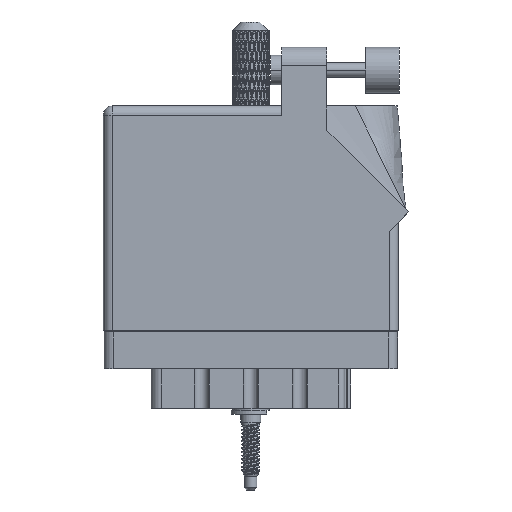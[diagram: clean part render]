
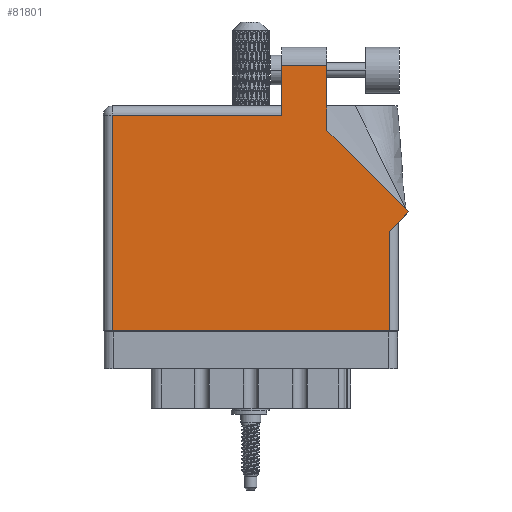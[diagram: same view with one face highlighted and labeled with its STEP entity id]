
A CAD part, front view. The second image highlights one B-rep face of the part: STEP entity #81801.
In plain terms, the highlighted face is planar.
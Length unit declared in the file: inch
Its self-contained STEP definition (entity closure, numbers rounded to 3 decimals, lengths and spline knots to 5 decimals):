
#190 = CARTESIAN_POINT ( 'NONE',  ( 1.524, 1.805, 0. ) ) ;
#552 = CARTESIAN_POINT ( 'NONE',  ( 0., 1.53, 0. ) ) ;
#3980 = ORIENTED_EDGE ( 'NONE', *, *, #29289, .T. ) ;
#4600 = LINE ( 'NONE', #6579, #17549 ) ;
#6579 = CARTESIAN_POINT ( 'NONE',  ( 0., 1.468, 0. ) ) ;
#6887 = DIRECTION ( 'NONE',  ( -0.707, 0.707, 0. ) ) ;
#7116 = DIRECTION ( 'NONE',  ( -1., 0., 0. ) ) ;
#8156 = DIRECTION ( 'NONE',  ( 0., 0., -1. ) ) ;
#11079 = LINE ( 'NONE', #96018, #40867 ) ;
#14745 = VECTOR ( 'NONE', #106330, 39.37008 ) ;
#15077 = VECTOR ( 'NONE', #34349, 39.37008 ) ;
#15244 = VERTEX_POINT ( 'NONE', #74955 ) ;
#16278 = CARTESIAN_POINT ( 'NONE',  ( 2.08071, 0.80771, 0. ) ) ;
#17549 = VECTOR ( 'NONE', #23921, 39.37008 ) ;
#20252 = EDGE_CURVE ( 'NONE', #39443, #98159, #63385, .T. ) ;
#22491 = CARTESIAN_POINT ( 'NONE',  ( 0.062, 0., 0. ) ) ;
#22607 = EDGE_CURVE ( 'NONE', #15244, #59050, #104486, .T. ) ;
#22668 = CARTESIAN_POINT ( 'NONE',  ( 1.948, 0., 0. ) ) ;
#23921 = DIRECTION ( 'NONE',  ( -1., 0., 0. ) ) ;
#25894 = VECTOR ( 'NONE', #74722, 39.37008 ) ;
#26081 = ORIENTED_EDGE ( 'NONE', *, *, #91178, .T. ) ;
#29289 = EDGE_CURVE ( 'NONE', #70744, #55007, #84373, .T. ) ;
#29454 = VERTEX_POINT ( 'NONE', #22668 ) ;
#32411 = CARTESIAN_POINT ( 'NONE',  ( 1.217, 1.805, 0. ) ) ;
#34349 = DIRECTION ( 'NONE',  ( 0., -1., 0. ) ) ;
#36263 = VERTEX_POINT ( 'NONE', #44023 ) ;
#36690 = LINE ( 'NONE', #73022, #14745 ) ;
#39443 = VERTEX_POINT ( 'NONE', #93223 ) ;
#40451 = VECTOR ( 'NONE', #42247, 39.37008 ) ;
#40867 = VECTOR ( 'NONE', #96360, 39.37008 ) ;
#42087 = ORIENTED_EDGE ( 'NONE', *, *, #47681, .T. ) ;
#42247 = DIRECTION ( 'NONE',  ( 0., 1., 0. ) ) ;
#42737 = CARTESIAN_POINT ( 'NONE',  ( 0.062, 0., 0. ) ) ;
#43338 = CARTESIAN_POINT ( 'NONE',  ( 1.524, 1.36442, 0. ) ) ;
#44023 = CARTESIAN_POINT ( 'NONE',  ( 1.217, 1.805, 0. ) ) ;
#44737 = EDGE_LOOP ( 'NONE', ( #3980, #26081, #102421, #78069, #91085, #100634, #42087, #61000, #99805 ) ) ;
#47681 = EDGE_CURVE ( 'NONE', #29454, #39443, #36690, .T. ) ;
#50270 = VECTOR ( 'NONE', #67216, 39.37008 ) ;
#55007 = VERTEX_POINT ( 'NONE', #190 ) ;
#57662 = LINE ( 'NONE', #100136, #15077 ) ;
#59050 = VERTEX_POINT ( 'NONE', #22491 ) ;
#60789 = LINE ( 'NONE', #32411, #69883 ) ;
#61000 = ORIENTED_EDGE ( 'NONE', *, *, #20252, .T. ) ;
#62182 = CARTESIAN_POINT ( 'NONE',  ( 1.524, 1.36442, 0. ) ) ;
#63385 = LINE ( 'NONE', #82721, #25894 ) ;
#67216 = DIRECTION ( 'NONE',  ( 0., -1., 0. ) ) ;
#69883 = VECTOR ( 'NONE', #7116, 39.37008 ) ;
#70744 = VERTEX_POINT ( 'NONE', #62182 ) ;
#71821 = EDGE_CURVE ( 'NONE', #77385, #15244, #4600, .T. ) ;
#73022 = CARTESIAN_POINT ( 'NONE',  ( 1.948, 0.737, 0. ) ) ;
#73121 = CARTESIAN_POINT ( 'NONE',  ( 1.217, 1.468, 0. ) ) ;
#73833 = DIRECTION ( 'NONE',  ( -1., 0., 0. ) ) ;
#74722 = DIRECTION ( 'NONE',  ( 0.707, 0.707, 0. ) ) ;
#74955 = CARTESIAN_POINT ( 'NONE',  ( 0.062, 1.468, 0. ) ) ;
#77385 = VERTEX_POINT ( 'NONE', #73121 ) ;
#78069 = ORIENTED_EDGE ( 'NONE', *, *, #71821, .T. ) ;
#81801 = ADVANCED_FACE ( 'NONE', ( #88837 ), #106779, .F. ) ;
#82721 = CARTESIAN_POINT ( 'NONE',  ( 2.01, 0.737, 0. ) ) ;
#82888 = EDGE_CURVE ( 'NONE', #59050, #29454, #11079, .T. ) ;
#84373 = LINE ( 'NONE', #43338, #40451 ) ;
#88837 = FACE_OUTER_BOUND ( 'NONE', #44737, .T. ) ;
#89478 = AXIS2_PLACEMENT_3D ( 'NONE', #552, #8156, #73833 ) ;
#91085 = ORIENTED_EDGE ( 'NONE', *, *, #22607, .T. ) ;
#91131 = VECTOR ( 'NONE', #6887, 39.37008 ) ;
#91178 = EDGE_CURVE ( 'NONE', #55007, #36263, #60789, .T. ) ;
#93223 = CARTESIAN_POINT ( 'NONE',  ( 1.948, 0.675, 0. ) ) ;
#93737 = LINE ( 'NONE', #16278, #91131 ) ;
#96018 = CARTESIAN_POINT ( 'NONE',  ( 0., 0., 0. ) ) ;
#96360 = DIRECTION ( 'NONE',  ( 1., 0., 0. ) ) ;
#96889 = EDGE_CURVE ( 'NONE', #36263, #77385, #57662, .T. ) ;
#97652 = EDGE_CURVE ( 'NONE', #98159, #70744, #93737, .T. ) ;
#98159 = VERTEX_POINT ( 'NONE', #101056 ) ;
#99805 = ORIENTED_EDGE ( 'NONE', *, *, #97652, .T. ) ;
#100136 = CARTESIAN_POINT ( 'NONE',  ( 1.217, 1.53, 0. ) ) ;
#100634 = ORIENTED_EDGE ( 'NONE', *, *, #82888, .T. ) ;
#101056 = CARTESIAN_POINT ( 'NONE',  ( 2.08071, 0.80771, 0. ) ) ;
#102421 = ORIENTED_EDGE ( 'NONE', *, *, #96889, .T. ) ;
#104486 = LINE ( 'NONE', #42737, #50270 ) ;
#106330 = DIRECTION ( 'NONE',  ( 0., 1., 0. ) ) ;
#106779 = PLANE ( 'NONE',  #89478 ) ;
